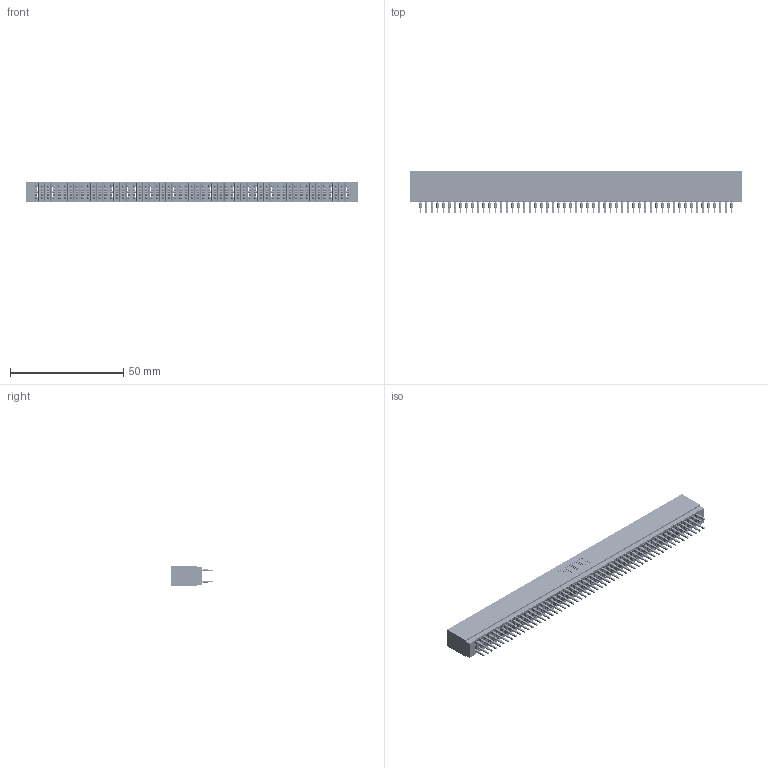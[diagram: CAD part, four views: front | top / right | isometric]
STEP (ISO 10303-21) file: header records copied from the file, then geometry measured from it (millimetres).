
FILE_DESCRIPTION (( 'STEP AP203' ), '1' );
FILE_NAME ('725-110-560-201.STEP', '2026-02-24T20:32:06', ( '' ), ( '' ), 'SwSTEP 2.0', 'SolidWorks 2023', '' );
FILE_SCHEMA (( 'CONFIG_CONTROL_DESIGN' ));
Products named in the file (3): 725 Part_Insulator Option - 01; 725-110-560-201; 745-292-001_560
Assembly tree (111 placements, depth 2):
  725-110-560-201
    725 Part_Insulator Option - 01
    745-292-001_560  x110
Bounding box: 146.3 x 18.8 x 8.89 mm (x, y, z)
Volume: 11942.9 mm3; surface area: 27237.4 mm2
Topology: 111 solids, 111 shells, 10930 faces, 29899 edges, 18978 vertices
Faces by surface type: plane 5665, cylinder 2405, bspline 2200, torus 660
Entity records: 91106 total; most frequent: CARTESIAN_POINT 16301, ORIENTED_EDGE 15762, DIRECTION 13765, EDGE_CURVE 7881, VECTOR 7361, LINE 7361, VERTEX_POINT 5026, AXIS2_PLACEMENT_3D 3202
